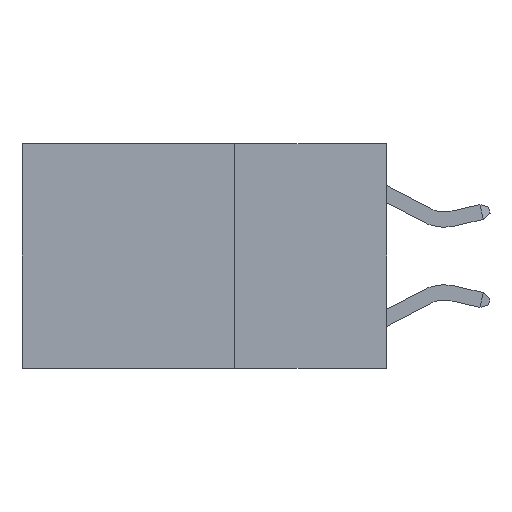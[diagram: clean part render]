
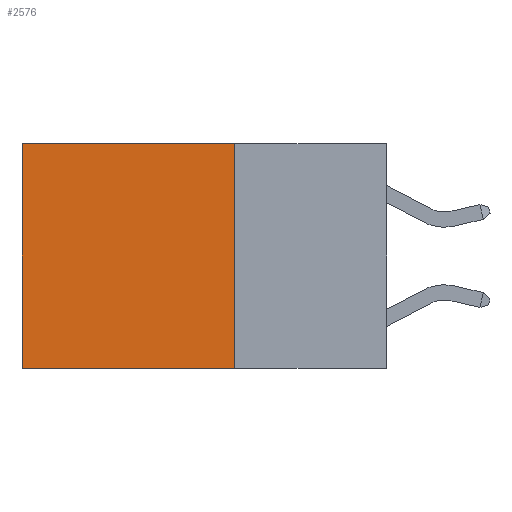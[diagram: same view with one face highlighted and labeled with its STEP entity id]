
A CAD part, left-side view. The second image highlights one B-rep face of the part: STEP entity #2576.
In plain terms, the highlighted planar face has unit normal (-1, 0, 0).
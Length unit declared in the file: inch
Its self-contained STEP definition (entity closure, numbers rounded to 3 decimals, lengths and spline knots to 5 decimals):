
#73 = VECTOR ( 'NONE', #14001, 39.37008 ) ;
#202 = LINE ( 'NONE', #2663, #12043 ) ;
#282 = EDGE_CURVE ( 'NONE', #10164, #4146, #202, .T. ) ;
#1101 = CARTESIAN_POINT ( 'NONE',  ( 0.2625, 0.25, 0. ) ) ;
#1352 = CARTESIAN_POINT ( 'NONE',  ( 0.2625, 0.25, -0.37 ) ) ;
#2112 = ORIENTED_EDGE ( 'NONE', *, *, #282, .T. ) ;
#2557 = EDGE_CURVE ( 'NONE', #4357, #10164, #6552, .T. ) ;
#2576 = ADVANCED_FACE ( 'NONE', ( #8877 ), #8258, .F. ) ;
#2663 = CARTESIAN_POINT ( 'NONE',  ( 0.2625, 0.6, 0. ) ) ;
#4146 = VERTEX_POINT ( 'NONE', #6505 ) ;
#4357 = VERTEX_POINT ( 'NONE', #1101 ) ;
#4513 = VERTEX_POINT ( 'NONE', #10542 ) ;
#4565 = CARTESIAN_POINT ( 'NONE',  ( 0.2625, 0.6, 0. ) ) ;
#5935 = DIRECTION ( 'NONE',  ( 0., 1., 0. ) ) ;
#5944 = DIRECTION ( 'NONE',  ( 0., 0., -1. ) ) ;
#5982 = DIRECTION ( 'NONE',  ( 0., 0., -1. ) ) ;
#6505 = CARTESIAN_POINT ( 'NONE',  ( 0.2625, 0.6, -0.37 ) ) ;
#6552 = LINE ( 'NONE', #10440, #11821 ) ;
#6750 = ORIENTED_EDGE ( 'NONE', *, *, #7948, .F. ) ;
#7306 = EDGE_CURVE ( 'NONE', #4513, #4146, #8277, .T. ) ;
#7570 = ORIENTED_EDGE ( 'NONE', *, *, #2557, .T. ) ;
#7948 = EDGE_CURVE ( 'NONE', #4357, #4513, #9336, .T. ) ;
#8258 = PLANE ( 'NONE',  #8401 ) ;
#8277 = LINE ( 'NONE', #1352, #10879 ) ;
#8401 = AXIS2_PLACEMENT_3D ( 'NONE', #10488, #12698, #5982 ) ;
#8877 = FACE_OUTER_BOUND ( 'NONE', #13150, .T. ) ;
#9336 = LINE ( 'NONE', #12917, #73 ) ;
#10164 = VERTEX_POINT ( 'NONE', #4565 ) ;
#10440 = CARTESIAN_POINT ( 'NONE',  ( 0.2625, 0.25, 0. ) ) ;
#10486 = DIRECTION ( 'NONE',  ( 0., 1., 0. ) ) ;
#10488 = CARTESIAN_POINT ( 'NONE',  ( 0.2625, 0.25, 0. ) ) ;
#10542 = CARTESIAN_POINT ( 'NONE',  ( 0.2625, 0.25, -0.37 ) ) ;
#10879 = VECTOR ( 'NONE', #10486, 39.37008 ) ;
#11821 = VECTOR ( 'NONE', #5935, 39.37008 ) ;
#12043 = VECTOR ( 'NONE', #5944, 39.37008 ) ;
#12698 = DIRECTION ( 'NONE',  ( 1., 0., 0. ) ) ;
#12917 = CARTESIAN_POINT ( 'NONE',  ( 0.2625, 0.25, 0. ) ) ;
#13150 = EDGE_LOOP ( 'NONE', ( #2112, #14484, #6750, #7570 ) ) ;
#14001 = DIRECTION ( 'NONE',  ( 0., 0., -1. ) ) ;
#14484 = ORIENTED_EDGE ( 'NONE', *, *, #7306, .F. ) ;
